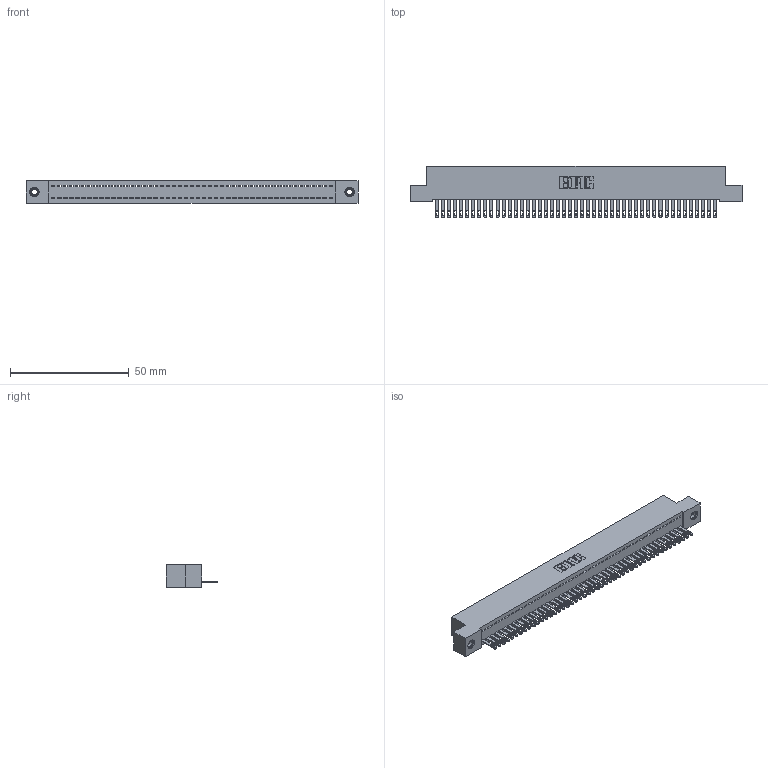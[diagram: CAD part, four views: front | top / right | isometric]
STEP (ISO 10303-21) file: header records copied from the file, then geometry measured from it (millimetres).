
FILE_DESCRIPTION (( 'STEP AP203' ), '1' );
FILE_NAME ('342-047-500-107.STEP', '2018-08-12T16:50:52', ( '' ), ( '' ), 'SwSTEP 2.0', 'SolidWorks 2016', '' );
FILE_SCHEMA (( 'CONFIG_CONTROL_DESIGN' ));
Length unit declared in the file: inch
Products named in the file (4): 342-047-500-107; 342 Part_TI; 345-292-001_345-293-100; 345-250-001_345-250-005-103
Assembly tree (50 placements, depth 2):
  342-047-500-107
    342 Part_TI
    345-292-001_345-293-100  x47
    345-250-001_345-250-005-103  x2
Bounding box: 139.7 x 21.85 x 9.4 mm (x, y, z)
Volume: 12283.7 mm3; surface area: 18256.2 mm2
Topology: 50 solids, 50 shells, 2708 faces, 8331 edges, 5546 vertices
Faces by surface type: plane 1790, cylinder 902, cone 12, torus 4
Entity records: 29070 total; most frequent: CARTESIAN_POINT 4994, ORIENTED_EDGE 4970, DIRECTION 4237, EDGE_CURVE 2485, LINE 2333, VECTOR 2333, VERTEX_POINT 1652, AXIS2_PLACEMENT_3D 952
